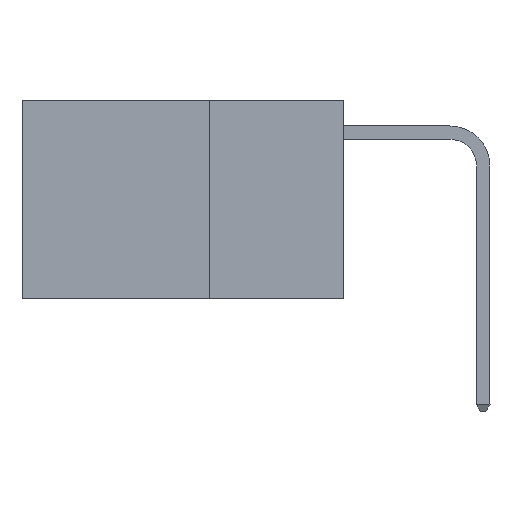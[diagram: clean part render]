
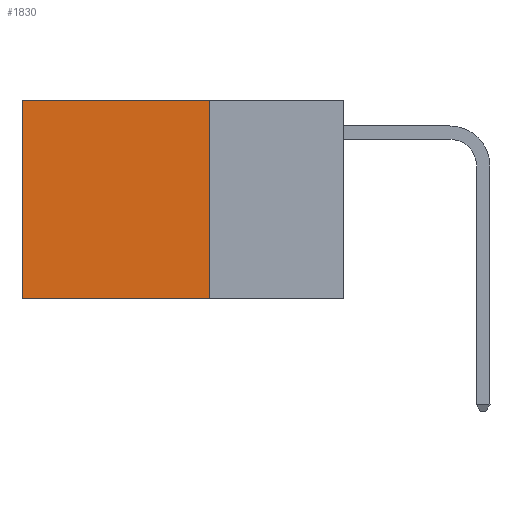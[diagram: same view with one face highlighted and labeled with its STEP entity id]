
A CAD part, left-side view. The second image highlights one B-rep face of the part: STEP entity #1830.
In plain terms, the highlighted planar face has unit normal (-1, 0, 0).
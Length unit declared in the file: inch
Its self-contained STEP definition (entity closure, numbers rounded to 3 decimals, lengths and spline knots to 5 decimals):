
#923 = CARTESIAN_POINT ( 'NONE',  ( 0.2625, 0.25, 0. ) ) ;
#1635 = DIRECTION ( 'NONE',  ( 1., 0., 0. ) ) ;
#1713 = LINE ( 'NONE', #11940, #10055 ) ;
#1731 = CARTESIAN_POINT ( 'NONE',  ( 0.2625, 0.6, -0.37 ) ) ;
#1830 = ADVANCED_FACE ( 'NONE', ( #8232 ), #8492, .F. ) ;
#2246 = ORIENTED_EDGE ( 'NONE', *, *, #4703, .F. ) ;
#3077 = VECTOR ( 'NONE', #12061, 39.37008 ) ;
#3324 = CARTESIAN_POINT ( 'NONE',  ( 0.2625, 0.6, 0. ) ) ;
#3327 = AXIS2_PLACEMENT_3D ( 'NONE', #7370, #1635, #9591 ) ;
#3794 = EDGE_CURVE ( 'NONE', #9332, #9676, #1713, .T. ) ;
#4059 = DIRECTION ( 'NONE',  ( 0., 1., 0. ) ) ;
#4154 = DIRECTION ( 'NONE',  ( 0., 0., -1. ) ) ;
#4703 = EDGE_CURVE ( 'NONE', #9676, #9724, #13763, .T. ) ;
#4955 = VECTOR ( 'NONE', #4059, 39.37008 ) ;
#6990 = LINE ( 'NONE', #14262, #9588 ) ;
#7370 = CARTESIAN_POINT ( 'NONE',  ( 0.2625, 0.25, 0. ) ) ;
#7466 = CARTESIAN_POINT ( 'NONE',  ( 0.2625, 0.25, -0.37 ) ) ;
#7787 = EDGE_LOOP ( 'NONE', ( #9711, #2246, #9337, #12815 ) ) ;
#8232 = FACE_OUTER_BOUND ( 'NONE', #7787, .T. ) ;
#8492 = PLANE ( 'NONE',  #3327 ) ;
#8534 = CARTESIAN_POINT ( 'NONE',  ( 0.2625, 0.25, -0.37 ) ) ;
#8795 = DIRECTION ( 'NONE',  ( 0., 1., 0. ) ) ;
#8800 = CARTESIAN_POINT ( 'NONE',  ( 0.2625, 0.6, 0. ) ) ;
#9072 = LINE ( 'NONE', #8800, #3077 ) ;
#9332 = VERTEX_POINT ( 'NONE', #923 ) ;
#9337 = ORIENTED_EDGE ( 'NONE', *, *, #3794, .F. ) ;
#9588 = VECTOR ( 'NONE', #8795, 39.37008 ) ;
#9591 = DIRECTION ( 'NONE',  ( 0., 0., -1. ) ) ;
#9676 = VERTEX_POINT ( 'NONE', #8534 ) ;
#9711 = ORIENTED_EDGE ( 'NONE', *, *, #12780, .T. ) ;
#9724 = VERTEX_POINT ( 'NONE', #1731 ) ;
#10055 = VECTOR ( 'NONE', #4154, 39.37008 ) ;
#10911 = VERTEX_POINT ( 'NONE', #3324 ) ;
#11940 = CARTESIAN_POINT ( 'NONE',  ( 0.2625, 0.25, 0. ) ) ;
#12061 = DIRECTION ( 'NONE',  ( 0., 0., -1. ) ) ;
#12780 = EDGE_CURVE ( 'NONE', #10911, #9724, #9072, .T. ) ;
#12815 = ORIENTED_EDGE ( 'NONE', *, *, #14065, .T. ) ;
#13763 = LINE ( 'NONE', #7466, #4955 ) ;
#14065 = EDGE_CURVE ( 'NONE', #9332, #10911, #6990, .T. ) ;
#14262 = CARTESIAN_POINT ( 'NONE',  ( 0.2625, 0.25, 0. ) ) ;
